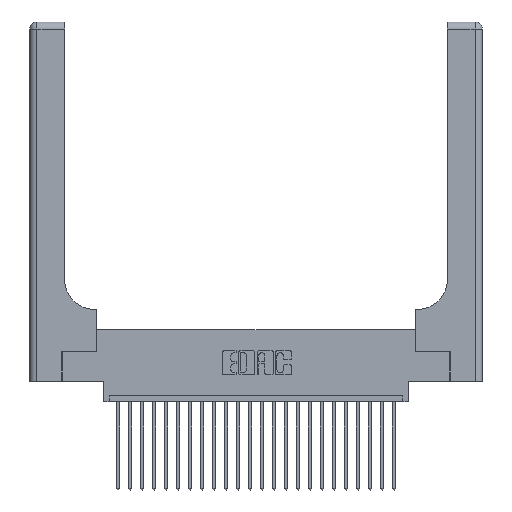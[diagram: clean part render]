
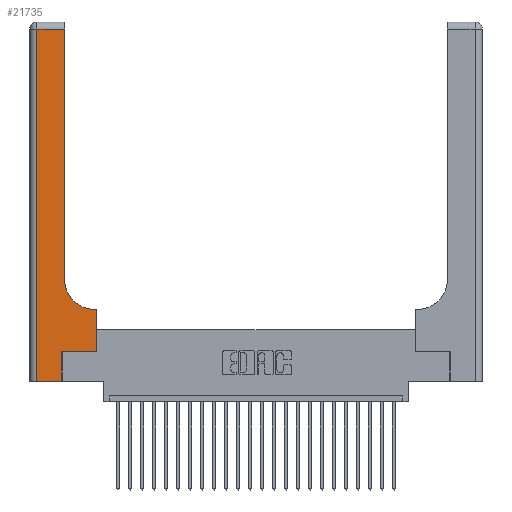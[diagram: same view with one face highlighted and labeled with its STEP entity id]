
A CAD part, top view. The second image highlights one B-rep face of the part: STEP entity #21735.
In plain terms, the highlighted planar face has unit normal (0, 0, 1).
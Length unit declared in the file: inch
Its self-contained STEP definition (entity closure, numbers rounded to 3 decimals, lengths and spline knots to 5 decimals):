
#65 = ORIENTED_EDGE ( 'NONE', *, *, #25556, .T. ) ;
#195 = CARTESIAN_POINT ( 'NONE',  ( 0.2915, 0.6, 0.37 ) ) ;
#284 = CARTESIAN_POINT ( 'NONE',  ( 0.269, 0., 0.37 ) ) ;
#528 = DIRECTION ( 'NONE',  ( -1., 0., 0. ) ) ;
#1096 = CARTESIAN_POINT ( 'NONE',  ( 0.2915, 2.94, 0.37 ) ) ;
#1183 = LINE ( 'NONE', #22581, #2119 ) ;
#1288 = DIRECTION ( 'NONE',  ( -1., 0., 0. ) ) ;
#1590 = EDGE_CURVE ( 'NONE', #7030, #23890, #7977, .T. ) ;
#2119 = VECTOR ( 'NONE', #14771, 39.37008 ) ;
#3159 = VECTOR ( 'NONE', #18145, 39.37008 ) ;
#3280 = DIRECTION ( 'NONE',  ( 0., 0., -1. ) ) ;
#3499 = CARTESIAN_POINT ( 'NONE',  ( 0.5585, 0.6, 0.37 ) ) ;
#3989 = CARTESIAN_POINT ( 'NONE',  ( 0.5415, 0.85, 0.37 ) ) ;
#4807 = LINE ( 'NONE', #18110, #6346 ) ;
#5061 = CARTESIAN_POINT ( 'NONE',  ( 0., 0., 0.37 ) ) ;
#5139 = DIRECTION ( 'NONE',  ( 0., 1., 0. ) ) ;
#5403 = CIRCLE ( 'NONE', #11265, 0.25 ) ;
#5717 = VERTEX_POINT ( 'NONE', #1096 ) ;
#6080 = ORIENTED_EDGE ( 'NONE', *, *, #23174, .T. ) ;
#6202 = DIRECTION ( 'NONE',  ( 0., 1., 0. ) ) ;
#6346 = VECTOR ( 'NONE', #6202, 39.37008 ) ;
#6469 = CARTESIAN_POINT ( 'NONE',  ( 0., 2.94, 0.37 ) ) ;
#6473 = LINE ( 'NONE', #17022, #16413 ) ;
#7030 = VERTEX_POINT ( 'NONE', #10166 ) ;
#7335 = EDGE_CURVE ( 'NONE', #15794, #10496, #23204, .T. ) ;
#7892 = ORIENTED_EDGE ( 'NONE', *, *, #25486, .T. ) ;
#7977 = LINE ( 'NONE', #5061, #23215 ) ;
#8013 = DIRECTION ( 'NONE',  ( 0., 0., -1. ) ) ;
#8567 = LINE ( 'NONE', #11622, #23156 ) ;
#9024 = EDGE_CURVE ( 'NONE', #12660, #7030, #8567, .T. ) ;
#10166 = CARTESIAN_POINT ( 'NONE',  ( 0.06, 0., 0.37 ) ) ;
#10496 = VERTEX_POINT ( 'NONE', #3499 ) ;
#10544 = ORIENTED_EDGE ( 'NONE', *, *, #9024, .T. ) ;
#11265 = AXIS2_PLACEMENT_3D ( 'NONE', #3989, #8013, #13743 ) ;
#11570 = ORIENTED_EDGE ( 'NONE', *, *, #19745, .T. ) ;
#11622 = CARTESIAN_POINT ( 'NONE',  ( 0.06, 3., 0.37 ) ) ;
#12608 = VECTOR ( 'NONE', #528, 39.37008 ) ;
#12660 = VERTEX_POINT ( 'NONE', #14023 ) ;
#12796 = ORIENTED_EDGE ( 'NONE', *, *, #7335, .T. ) ;
#13743 = DIRECTION ( 'NONE',  ( 1., 0., 0. ) ) ;
#14013 = VERTEX_POINT ( 'NONE', #15985 ) ;
#14023 = CARTESIAN_POINT ( 'NONE',  ( 0.06, 2.94, 0.37 ) ) ;
#14049 = DIRECTION ( 'NONE',  ( 0., -1., 0. ) ) ;
#14771 = DIRECTION ( 'NONE',  ( 1., 0., 0. ) ) ;
#15667 = LINE ( 'NONE', #6469, #12608 ) ;
#15755 = ORIENTED_EDGE ( 'NONE', *, *, #23981, .T. ) ;
#15794 = VERTEX_POINT ( 'NONE', #24074 ) ;
#15985 = CARTESIAN_POINT ( 'NONE',  ( 0.5415, 0.6, 0.37 ) ) ;
#16413 = VECTOR ( 'NONE', #5139, 39.37008 ) ;
#16989 = FACE_OUTER_BOUND ( 'NONE', #22975, .T. ) ;
#17022 = CARTESIAN_POINT ( 'NONE',  ( 0.269, 0., 0.37 ) ) ;
#17220 = CARTESIAN_POINT ( 'NONE',  ( 0.269, 0.25, 0.37 ) ) ;
#18110 = CARTESIAN_POINT ( 'NONE',  ( 0.2915, 3., 0.37 ) ) ;
#18145 = DIRECTION ( 'NONE',  ( -1., 0., 0. ) ) ;
#18253 = DIRECTION ( 'NONE',  ( 0., 1., 0. ) ) ;
#18806 = DIRECTION ( 'NONE',  ( 1., 0., 0. ) ) ;
#18924 = ORIENTED_EDGE ( 'NONE', *, *, #21099, .T. ) ;
#18998 = VERTEX_POINT ( 'NONE', #21737 ) ;
#19378 = CARTESIAN_POINT ( 'NONE',  ( 0., 3., 0.37 ) ) ;
#19745 = EDGE_CURVE ( 'NONE', #22898, #15794, #1183, .T. ) ;
#21099 = EDGE_CURVE ( 'NONE', #23890, #22898, #6473, .T. ) ;
#21735 = ADVANCED_FACE ( 'NONE', ( #16989 ), #25406, .F. ) ;
#21737 = CARTESIAN_POINT ( 'NONE',  ( 0.2915, 0.85, 0.37 ) ) ;
#22581 = CARTESIAN_POINT ( 'NONE',  ( 0.269, 0.25, 0.37 ) ) ;
#22784 = LINE ( 'NONE', #195, #3159 ) ;
#22898 = VERTEX_POINT ( 'NONE', #17220 ) ;
#22975 = EDGE_LOOP ( 'NONE', ( #7892, #65, #10544, #25218, #18924, #11570, #12796, #15755, #6080 ) ) ;
#23156 = VECTOR ( 'NONE', #14049, 39.37008 ) ;
#23174 = EDGE_CURVE ( 'NONE', #14013, #18998, #5403, .T. ) ;
#23204 = LINE ( 'NONE', #24098, #25403 ) ;
#23215 = VECTOR ( 'NONE', #18806, 39.37008 ) ;
#23890 = VERTEX_POINT ( 'NONE', #284 ) ;
#23981 = EDGE_CURVE ( 'NONE', #10496, #14013, #22784, .T. ) ;
#24074 = CARTESIAN_POINT ( 'NONE',  ( 0.5585, 0.25, 0.37 ) ) ;
#24098 = CARTESIAN_POINT ( 'NONE',  ( 0.5585, 0.25, 0.37 ) ) ;
#24408 = AXIS2_PLACEMENT_3D ( 'NONE', #19378, #3280, #1288 ) ;
#25218 = ORIENTED_EDGE ( 'NONE', *, *, #1590, .T. ) ;
#25403 = VECTOR ( 'NONE', #18253, 39.37008 ) ;
#25406 = PLANE ( 'NONE',  #24408 ) ;
#25486 = EDGE_CURVE ( 'NONE', #18998, #5717, #4807, .T. ) ;
#25556 = EDGE_CURVE ( 'NONE', #5717, #12660, #15667, .T. ) ;
